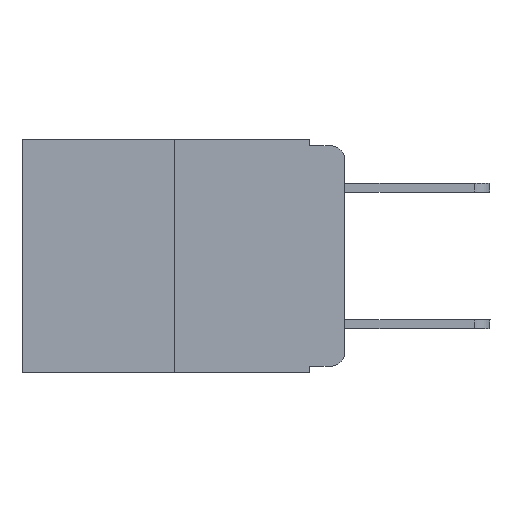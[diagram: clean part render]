
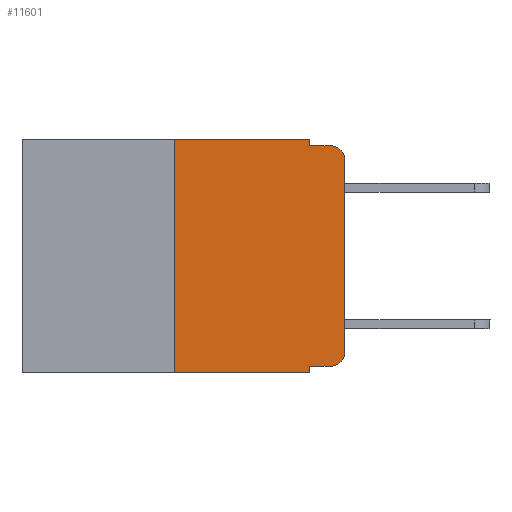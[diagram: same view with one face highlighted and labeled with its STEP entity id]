
A CAD part, left-side view. The second image highlights one B-rep face of the part: STEP entity #11601.
In plain terms, the highlighted planar face has unit normal (-1, 0, 0).
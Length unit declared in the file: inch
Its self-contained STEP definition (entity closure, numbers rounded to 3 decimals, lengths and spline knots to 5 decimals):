
#617 = CARTESIAN_POINT ( 'NONE',  ( 0., 0.473, -0.343 ) ) ;
#778 = EDGE_CURVE ( 'NONE', #1319, #16586, #10885, .T. ) ;
#1212 = VERTEX_POINT ( 'NONE', #18489 ) ;
#1319 = VERTEX_POINT ( 'NONE', #17323 ) ;
#1696 = EDGE_CURVE ( 'NONE', #11586, #1212, #16712, .T. ) ;
#1714 = CARTESIAN_POINT ( 'NONE',  ( 0., 0.25, 0. ) ) ;
#2437 = ORIENTED_EDGE ( 'NONE', *, *, #7860, .T. ) ;
#2800 = AXIS2_PLACEMENT_3D ( 'NONE', #3019, #9304, #20011 ) ;
#3019 = CARTESIAN_POINT ( 'NONE',  ( 0., 0.02, -0.313 ) ) ;
#3169 = CARTESIAN_POINT ( 'NONE',  ( 0., 0.02, -0.03 ) ) ;
#3326 = VECTOR ( 'NONE', #8250, 39.37008 ) ;
#4151 = CARTESIAN_POINT ( 'NONE',  ( 0., 0.25, 0. ) ) ;
#4303 = CARTESIAN_POINT ( 'NONE',  ( 0., 0., -0.313 ) ) ;
#4329 = VECTOR ( 'NONE', #9763, 39.37008 ) ;
#4376 = CIRCLE ( 'NONE', #17873, 0.02 ) ;
#4577 = ORIENTED_EDGE ( 'NONE', *, *, #17924, .F. ) ;
#4606 = DIRECTION ( 'NONE',  ( 0., 0., -1. ) ) ;
#4883 = DIRECTION ( 'NONE',  ( 1., 0., 0. ) ) ;
#4961 = VERTEX_POINT ( 'NONE', #1714 ) ;
#5306 = CARTESIAN_POINT ( 'NONE',  ( 0., 0., 0. ) ) ;
#5900 = ORIENTED_EDGE ( 'NONE', *, *, #16588, .T. ) ;
#6008 = CARTESIAN_POINT ( 'NONE',  ( 0., 0.25, -0.343 ) ) ;
#6074 = VERTEX_POINT ( 'NONE', #8695 ) ;
#6116 = EDGE_CURVE ( 'NONE', #8363, #18575, #6162, .T. ) ;
#6162 = LINE ( 'NONE', #5306, #17092 ) ;
#6460 = DIRECTION ( 'NONE',  ( -1., 0., 0. ) ) ;
#7234 = EDGE_LOOP ( 'NONE', ( #14113, #8516, #9664, #12514, #4577, #7997, #5900, #13534, #17925, #2437 ) ) ;
#7313 = VERTEX_POINT ( 'NONE', #19477 ) ;
#7860 = EDGE_CURVE ( 'NONE', #6074, #8363, #8832, .T. ) ;
#7997 = ORIENTED_EDGE ( 'NONE', *, *, #11346, .F. ) ;
#8250 = DIRECTION ( 'NONE',  ( 0., 0., -1. ) ) ;
#8363 = VERTEX_POINT ( 'NONE', #4303 ) ;
#8458 = CARTESIAN_POINT ( 'NONE',  ( 0., 0.051, -0.343 ) ) ;
#8516 = ORIENTED_EDGE ( 'NONE', *, *, #11542, .T. ) ;
#8695 = CARTESIAN_POINT ( 'NONE',  ( 0., 0.02, -0.333 ) ) ;
#8832 = CIRCLE ( 'NONE', #2800, 0.02 ) ;
#8885 = AXIS2_PLACEMENT_3D ( 'NONE', #14037, #4883, #4606 ) ;
#9056 = EDGE_CURVE ( 'NONE', #1319, #6074, #18470, .T. ) ;
#9114 = LINE ( 'NONE', #16317, #20022 ) ;
#9304 = DIRECTION ( 'NONE',  ( -1., 0., 0. ) ) ;
#9473 = CARTESIAN_POINT ( 'NONE',  ( 0., 0.051, 0. ) ) ;
#9664 = ORIENTED_EDGE ( 'NONE', *, *, #14466, .F. ) ;
#9763 = DIRECTION ( 'NONE',  ( 0., 0., -1. ) ) ;
#9813 = CARTESIAN_POINT ( 'NONE',  ( 0., 0.051, 0. ) ) ;
#9914 = VECTOR ( 'NONE', #19233, 39.37008 ) ;
#10885 = LINE ( 'NONE', #14414, #4329 ) ;
#11346 = EDGE_CURVE ( 'NONE', #17498, #4961, #15810, .T. ) ;
#11542 = EDGE_CURVE ( 'NONE', #18575, #7313, #4376, .T. ) ;
#11586 = VERTEX_POINT ( 'NONE', #9473 ) ;
#11601 = ADVANCED_FACE ( 'NONE', ( #13586 ), #18750, .F. ) ;
#12092 = DIRECTION ( 'NONE',  ( 0., -1., 0. ) ) ;
#12514 = ORIENTED_EDGE ( 'NONE', *, *, #1696, .F. ) ;
#13113 = DIRECTION ( 'NONE',  ( 0., -1., 0. ) ) ;
#13534 = ORIENTED_EDGE ( 'NONE', *, *, #778, .F. ) ;
#13586 = FACE_OUTER_BOUND ( 'NONE', #7234, .T. ) ;
#13816 = VECTOR ( 'NONE', #19897, 39.37008 ) ;
#14037 = CARTESIAN_POINT ( 'NONE',  ( 0., 0.473, 0. ) ) ;
#14113 = ORIENTED_EDGE ( 'NONE', *, *, #6116, .T. ) ;
#14414 = CARTESIAN_POINT ( 'NONE',  ( 0., 0.051, 0. ) ) ;
#14466 = EDGE_CURVE ( 'NONE', #1212, #7313, #17126, .T. ) ;
#14876 = DIRECTION ( 'NONE',  ( 0., 0., 1. ) ) ;
#15487 = CARTESIAN_POINT ( 'NONE',  ( 0., 0.051, -0.01 ) ) ;
#15579 = VECTOR ( 'NONE', #14876, 39.37008 ) ;
#15810 = LINE ( 'NONE', #4151, #15579 ) ;
#15955 = CARTESIAN_POINT ( 'NONE',  ( 0., 0., -0.03 ) ) ;
#16148 = DIRECTION ( 'NONE',  ( 0., 0., 1. ) ) ;
#16317 = CARTESIAN_POINT ( 'NONE',  ( 0., 0.473, 0. ) ) ;
#16586 = VERTEX_POINT ( 'NONE', #8458 ) ;
#16588 = EDGE_CURVE ( 'NONE', #17498, #16586, #16923, .T. ) ;
#16712 = LINE ( 'NONE', #9813, #3326 ) ;
#16781 = CARTESIAN_POINT ( 'NONE',  ( 0., 0.051, -0.333 ) ) ;
#16923 = LINE ( 'NONE', #617, #9914 ) ;
#17092 = VECTOR ( 'NONE', #16148, 39.37008 ) ;
#17126 = LINE ( 'NONE', #15487, #19576 ) ;
#17323 = CARTESIAN_POINT ( 'NONE',  ( 0., 0.051, -0.333 ) ) ;
#17498 = VERTEX_POINT ( 'NONE', #6008 ) ;
#17873 = AXIS2_PLACEMENT_3D ( 'NONE', #3169, #6460, #18878 ) ;
#17924 = EDGE_CURVE ( 'NONE', #4961, #11586, #9114, .T. ) ;
#17925 = ORIENTED_EDGE ( 'NONE', *, *, #9056, .T. ) ;
#18470 = LINE ( 'NONE', #16781, #13816 ) ;
#18489 = CARTESIAN_POINT ( 'NONE',  ( 0., 0.051, -0.01 ) ) ;
#18575 = VERTEX_POINT ( 'NONE', #15955 ) ;
#18750 = PLANE ( 'NONE',  #8885 ) ;
#18878 = DIRECTION ( 'NONE',  ( 0., 0., -1. ) ) ;
#19233 = DIRECTION ( 'NONE',  ( 0., -1., 0. ) ) ;
#19477 = CARTESIAN_POINT ( 'NONE',  ( 0., 0.02, -0.01 ) ) ;
#19576 = VECTOR ( 'NONE', #12092, 39.37008 ) ;
#19897 = DIRECTION ( 'NONE',  ( 0., -1., 0. ) ) ;
#20011 = DIRECTION ( 'NONE',  ( 0., 0., -1. ) ) ;
#20022 = VECTOR ( 'NONE', #13113, 39.37008 ) ;
